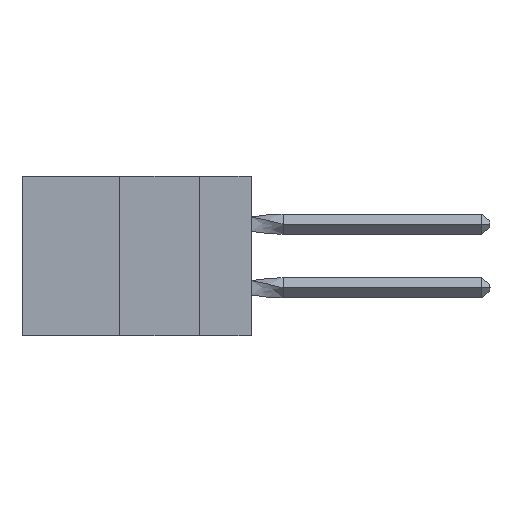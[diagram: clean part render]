
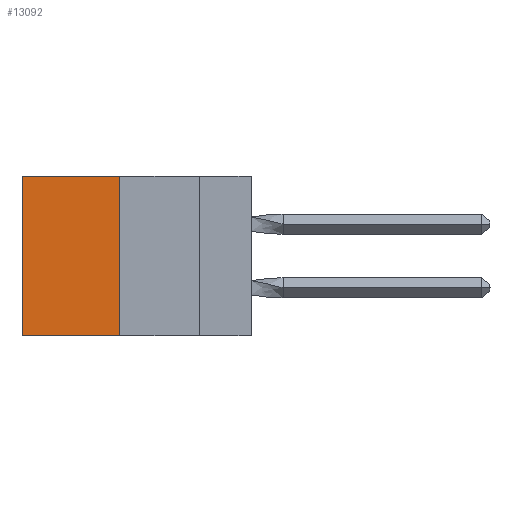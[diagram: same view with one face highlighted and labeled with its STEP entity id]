
A CAD part, left-side view. The second image highlights one B-rep face of the part: STEP entity #13092.
In plain terms, the highlighted planar face has unit normal (-1, 0, 0).
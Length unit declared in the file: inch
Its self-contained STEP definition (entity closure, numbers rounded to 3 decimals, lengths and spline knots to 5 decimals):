
#454 = LINE ( 'NONE', #17029, #7870 ) ;
#976 = DIRECTION ( 'NONE',  ( 0., 0., -1. ) ) ;
#2528 = LINE ( 'NONE', #22878, #6529 ) ;
#3247 = VECTOR ( 'NONE', #976, 39.37008 ) ;
#3256 = VERTEX_POINT ( 'NONE', #18047 ) ;
#3529 = VERTEX_POINT ( 'NONE', #3661 ) ;
#3661 = CARTESIAN_POINT ( 'NONE',  ( 0.305, 0.72, 0. ) ) ;
#4033 = LINE ( 'NONE', #17121, #16592 ) ;
#4702 = VERTEX_POINT ( 'NONE', #14474 ) ;
#5378 = DIRECTION ( 'NONE',  ( 0., 0., -1. ) ) ;
#6250 = ORIENTED_EDGE ( 'NONE', *, *, #17554, .T. ) ;
#6529 = VECTOR ( 'NONE', #5378, 39.37008 ) ;
#6889 = PLANE ( 'NONE',  #25150 ) ;
#7870 = VECTOR ( 'NONE', #19101, 39.37008 ) ;
#8414 = VERTEX_POINT ( 'NONE', #18342 ) ;
#11254 = EDGE_CURVE ( 'NONE', #3256, #3529, #454, .T. ) ;
#12753 = CARTESIAN_POINT ( 'NONE',  ( 0.305, 0.72, -0.5 ) ) ;
#13092 = ADVANCED_FACE ( 'NONE', ( #16991 ), #6889, .F. ) ;
#14474 = CARTESIAN_POINT ( 'NONE',  ( 0.305, 0.413, -0.5 ) ) ;
#14630 = EDGE_CURVE ( 'NONE', #4702, #8414, #4033, .T. ) ;
#14699 = ORIENTED_EDGE ( 'NONE', *, *, #23354, .F. ) ;
#14780 = ORIENTED_EDGE ( 'NONE', *, *, #11254, .T. ) ;
#16592 = VECTOR ( 'NONE', #23091, 39.37008 ) ;
#16991 = FACE_OUTER_BOUND ( 'NONE', #19914, .T. ) ;
#17029 = CARTESIAN_POINT ( 'NONE',  ( 0.305, 0.413, 0. ) ) ;
#17121 = CARTESIAN_POINT ( 'NONE',  ( 0.305, 0.413, -0.5 ) ) ;
#17554 = EDGE_CURVE ( 'NONE', #3529, #8414, #22899, .T. ) ;
#18047 = CARTESIAN_POINT ( 'NONE',  ( 0.305, 0.413, 0. ) ) ;
#18342 = CARTESIAN_POINT ( 'NONE',  ( 0.305, 0.72, -0.5 ) ) ;
#19101 = DIRECTION ( 'NONE',  ( 0., 1., 0. ) ) ;
#19914 = EDGE_LOOP ( 'NONE', ( #6250, #22511, #14699, #14780 ) ) ;
#20526 = DIRECTION ( 'NONE',  ( 0., 0., -1. ) ) ;
#22482 = DIRECTION ( 'NONE',  ( 1., 0., 0. ) ) ;
#22511 = ORIENTED_EDGE ( 'NONE', *, *, #14630, .F. ) ;
#22878 = CARTESIAN_POINT ( 'NONE',  ( 0.305, 0.413, -0.5 ) ) ;
#22899 = LINE ( 'NONE', #12753, #3247 ) ;
#23091 = DIRECTION ( 'NONE',  ( 0., 1., 0. ) ) ;
#23354 = EDGE_CURVE ( 'NONE', #3256, #4702, #2528, .T. ) ;
#24551 = CARTESIAN_POINT ( 'NONE',  ( 0.305, 0.413, -0.5 ) ) ;
#25150 = AXIS2_PLACEMENT_3D ( 'NONE', #24551, #22482, #20526 ) ;
